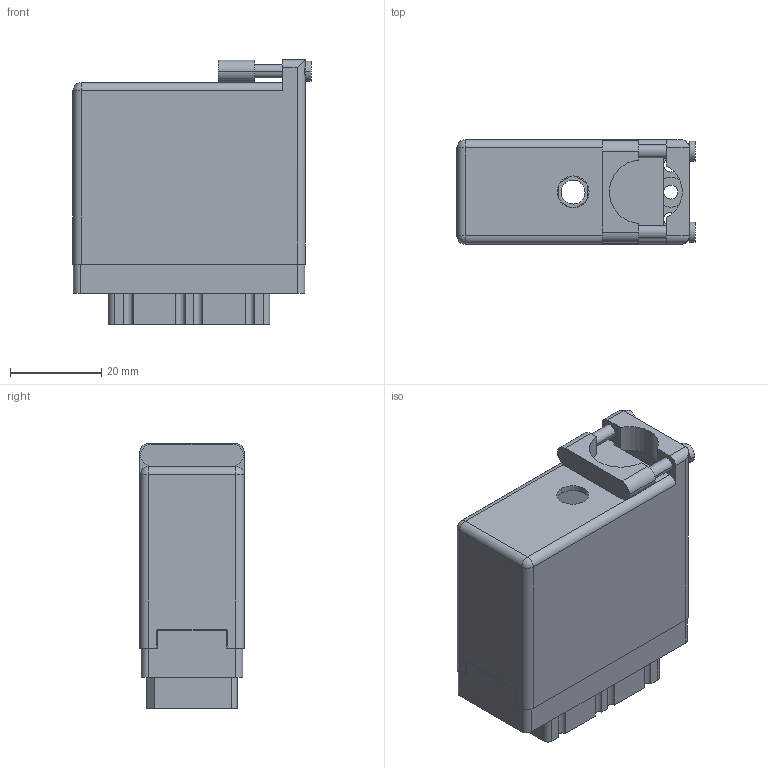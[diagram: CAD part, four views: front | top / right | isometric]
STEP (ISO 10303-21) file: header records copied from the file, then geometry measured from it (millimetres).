
FILE_DESCRIPTION (( 'STEP AP203' ), '1' );
FILE_NAME ('519-036-000-460.STEP', '2020-09-09T20:06:19', ( '' ), ( '' ), 'SwSTEP 2.0', 'SolidWorks 2020', '' );
FILE_SCHEMA (( 'CONFIG_CONTROL_DESIGN' ));
Length unit declared in the file: inch
Products named in the file (3): 516-230-001_Metal - 038 Top Entry; 519-036-000-460; 519 Receptacle Insulator_036
Assembly tree (2 placements, depth 2):
  519-036-000-460
    519 Receptacle Insulator_036
    516-230-001_Metal - 038 Top Entry
Bounding box: 52.27 x 22.83 x 58.09 mm (x, y, z)
Volume: 20139.2 mm3; surface area: 28157.6 mm2
Topology: 2 solids, 2 shells, 910 faces, 2659 edges, 1766 vertices
Faces by surface type: plane 644, cylinder 262, cone 2, sphere 2
Entity records: 30652 total; most frequent: CARTESIAN_POINT 5380, ORIENTED_EDGE 5314, DIRECTION 5149, EDGE_CURVE 2657, LINE 1983, VECTOR 1983, VERTEX_POINT 1766, AXIS2_PLACEMENT_3D 1583
